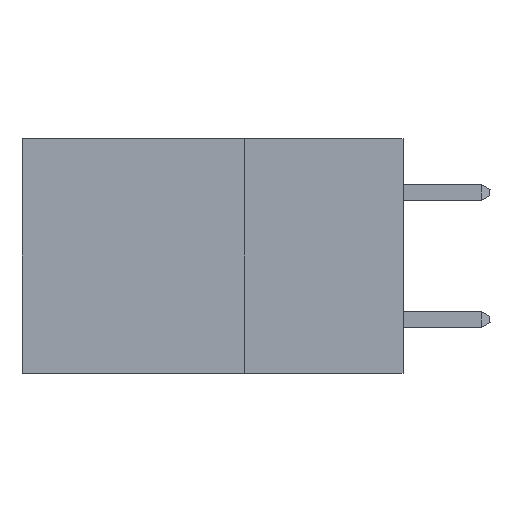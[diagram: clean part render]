
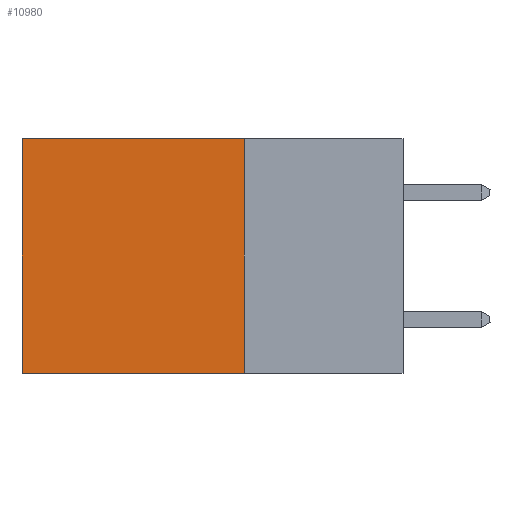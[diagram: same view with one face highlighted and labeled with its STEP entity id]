
A CAD part, left-side view. The second image highlights one B-rep face of the part: STEP entity #10980.
In plain terms, the highlighted planar face has unit normal (-1, 0, 0).
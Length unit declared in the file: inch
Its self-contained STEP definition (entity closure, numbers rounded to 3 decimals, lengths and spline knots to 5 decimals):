
#171 = VECTOR ( 'NONE', #7567, 39.37008 ) ;
#698 = VERTEX_POINT ( 'NONE', #5060 ) ;
#895 = EDGE_CURVE ( 'NONE', #6712, #10215, #1000, .T. ) ;
#1000 = LINE ( 'NONE', #4857, #13232 ) ;
#1452 = VECTOR ( 'NONE', #4086, 39.37008 ) ;
#1494 = DIRECTION ( 'NONE',  ( 0., 0., -1. ) ) ;
#1800 = CARTESIAN_POINT ( 'NONE',  ( 0.2875, 0.6, 0. ) ) ;
#3006 = CARTESIAN_POINT ( 'NONE',  ( 0.2875, 0.25, 0. ) ) ;
#3571 = CARTESIAN_POINT ( 'NONE',  ( 0.2875, 0.25, -0.37 ) ) ;
#3795 = EDGE_CURVE ( 'NONE', #698, #6712, #7921, .T. ) ;
#3800 = ORIENTED_EDGE ( 'NONE', *, *, #12343, .F. ) ;
#3918 = LINE ( 'NONE', #8661, #171 ) ;
#4086 = DIRECTION ( 'NONE',  ( 0., 1., 0. ) ) ;
#4857 = CARTESIAN_POINT ( 'NONE',  ( 0.2875, 0.6, 0. ) ) ;
#5060 = CARTESIAN_POINT ( 'NONE',  ( 0.2875, 0.25, 0. ) ) ;
#5445 = PLANE ( 'NONE',  #11351 ) ;
#6034 = EDGE_LOOP ( 'NONE', ( #9116, #3800, #12821, #11882 ) ) ;
#6378 = DIRECTION ( 'NONE',  ( 1., 0., 0. ) ) ;
#6712 = VERTEX_POINT ( 'NONE', #1800 ) ;
#7234 = CARTESIAN_POINT ( 'NONE',  ( 0.2875, 0.6, -0.37 ) ) ;
#7502 = DIRECTION ( 'NONE',  ( 0., 0., -1. ) ) ;
#7567 = DIRECTION ( 'NONE',  ( 0., 0., -1. ) ) ;
#7921 = LINE ( 'NONE', #3006, #1452 ) ;
#8001 = EDGE_CURVE ( 'NONE', #698, #12895, #3918, .T. ) ;
#8661 = CARTESIAN_POINT ( 'NONE',  ( 0.2875, 0.25, 0. ) ) ;
#9116 = ORIENTED_EDGE ( 'NONE', *, *, #895, .T. ) ;
#9138 = DIRECTION ( 'NONE',  ( 0., 1., 0. ) ) ;
#9415 = LINE ( 'NONE', #3571, #13111 ) ;
#10215 = VERTEX_POINT ( 'NONE', #7234 ) ;
#10980 = ADVANCED_FACE ( 'NONE', ( #12982 ), #5445, .F. ) ;
#11063 = CARTESIAN_POINT ( 'NONE',  ( 0.2875, 0.25, -0.37 ) ) ;
#11351 = AXIS2_PLACEMENT_3D ( 'NONE', #12893, #6378, #7502 ) ;
#11882 = ORIENTED_EDGE ( 'NONE', *, *, #3795, .T. ) ;
#12343 = EDGE_CURVE ( 'NONE', #12895, #10215, #9415, .T. ) ;
#12821 = ORIENTED_EDGE ( 'NONE', *, *, #8001, .F. ) ;
#12893 = CARTESIAN_POINT ( 'NONE',  ( 0.2875, 0.25, 0. ) ) ;
#12895 = VERTEX_POINT ( 'NONE', #11063 ) ;
#12982 = FACE_OUTER_BOUND ( 'NONE', #6034, .T. ) ;
#13111 = VECTOR ( 'NONE', #9138, 39.37008 ) ;
#13232 = VECTOR ( 'NONE', #1494, 39.37008 ) ;
